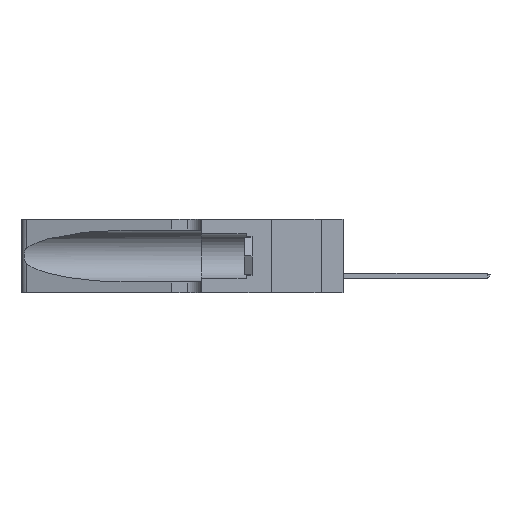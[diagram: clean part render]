
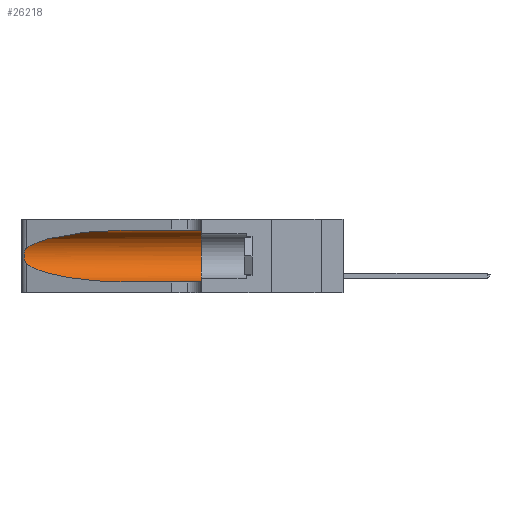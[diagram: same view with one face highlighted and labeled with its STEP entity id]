
A CAD part, left-side view. The second image highlights one B-rep face of the part: STEP entity #26218.
In plain terms, the highlighted cylindrical face has radius 3.308 mm (diameter 6.617 mm), a partial arc.
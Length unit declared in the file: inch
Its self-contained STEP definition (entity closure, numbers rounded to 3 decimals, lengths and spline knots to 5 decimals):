
#299 = LINE ( 'NONE', #27840, #22254 ) ;
#652 = CARTESIAN_POINT ( 'NONE',  ( 0.25487, 1.22718, 0.22369 ) ) ;
#789 = CARTESIAN_POINT ( 'NONE',  ( 0.25854, 1.2359, 0.20912 ) ) ;
#1079 = CARTESIAN_POINT ( 'NONE',  ( 0.25789, 1.23486, 0.15765 ) ) ;
#1167 = EDGE_CURVE ( 'NONE', #31608, #3406, #10031, .T. ) ;
#2053 = CARTESIAN_POINT ( 'NONE',  ( 0.18966, 0.96281, 0.31525 ) ) ;
#2174 = VERTEX_POINT ( 'NONE', #25149 ) ;
#3406 = VERTEX_POINT ( 'NONE', #5205 ) ;
#3571 = LINE ( 'NONE', #37456, #24119 ) ;
#3622 = ORIENTED_EDGE ( 'NONE', *, *, #30223, .T. ) ;
#5205 = CARTESIAN_POINT ( 'NONE',  ( 0.25487, 1.22718, 0.22369 ) ) ;
#6838 = CARTESIAN_POINT ( 'NONE',  ( 0.26018, 1.23835, 0.19895 ) ) ;
#7117 = CARTESIAN_POINT ( 'NONE',  ( 0.25787, 1.23484, 0.2124 ) ) ;
#7829 = VERTEX_POINT ( 'NONE', #31679 ) ;
#9673 = DIRECTION ( 'NONE',  ( 0., 0., 1. ) ) ;
#10031 =( BOUNDED_CURVE ( )  B_SPLINE_CURVE ( 3, ( #25748, #2053, #31788, #22376 ),
 .UNSPECIFIED., .F., .F. ) 
 B_SPLINE_CURVE_WITH_KNOTS ( ( 4, 4 ),
 ( 1.5708, 2.84003 ),
 .UNSPECIFIED. ) 
 CURVE ( )  GEOMETRIC_REPRESENTATION_ITEM ( )  RATIONAL_B_SPLINE_CURVE ( ( 1., 0.87, 0.87, 1. ) ) 
 REPRESENTATION_ITEM ( '' )  );
#11301 = CARTESIAN_POINT ( 'NONE',  ( 0.1305, 0.72297, 0.31525 ) ) ;
#11397 = ORIENTED_EDGE ( 'NONE', *, *, #26656, .F. ) ;
#11988 = AXIS2_PLACEMENT_3D ( 'NONE', #27702, #15833, #18851 ) ;
#12249 = CARTESIAN_POINT ( 'NONE',  ( 0.1305, 0.35, 0.05475 ) ) ;
#12529 = EDGE_CURVE ( 'NONE', #31608, #7829, #3571, .T. ) ;
#12671 = CARTESIAN_POINT ( 'NONE',  ( 0.25487, 1.22718, 0.14631 ) ) ;
#13066 = CARTESIAN_POINT ( 'NONE',  ( 0.25639, 1.23184, 0.21858 ) ) ;
#13346 = ORIENTED_EDGE ( 'NONE', *, *, #20162, .T. ) ;
#15113 = VERTEX_POINT ( 'NONE', #12249 ) ;
#15776 = CARTESIAN_POINT ( 'NONE',  ( 0.25856, 1.23593, 0.16098 ) ) ;
#15833 = DIRECTION ( 'NONE',  ( 0., -1., 0. ) ) ;
#16363 = CARTESIAN_POINT ( 'NONE',  ( 0.25487, 1.22718, 0.14631 ) ) ;
#16800 = FACE_OUTER_BOUND ( 'NONE', #24280, .T. ) ;
#18458 = DIRECTION ( 'NONE',  ( 0., 1., 0. ) ) ;
#18851 = DIRECTION ( 'NONE',  ( 0., 0., -1. ) ) ;
#19059 = CARTESIAN_POINT ( 'NONE',  ( 0.25639, 1.23186, 0.15144 ) ) ;
#19532 = DIRECTION ( 'NONE',  ( 0., -1., 0. ) ) ;
#20162 = EDGE_CURVE ( 'NONE', #2174, #15113, #299, .T. ) ;
#20496 = AXIS2_PLACEMENT_3D ( 'NONE', #24338, #18458, #9673 ) ;
#21499 = CARTESIAN_POINT ( 'NONE',  ( 0.26017, 1.23833, 0.17102 ) ) ;
#21636 = CARTESIAN_POINT ( 'NONE',  ( 0.25555, 1.22993, 0.14849 ) ) ;
#22254 = VECTOR ( 'NONE', #36480, 39.37008 ) ;
#22376 = CARTESIAN_POINT ( 'NONE',  ( 0.25487, 1.22718, 0.22369 ) ) ;
#23088 = CARTESIAN_POINT ( 'NONE',  ( 0.1305, 0.72297, 0.05475 ) ) ;
#23258 = ORIENTED_EDGE ( 'NONE', *, *, #35990, .T. ) ;
#23389 = VERTEX_POINT ( 'NONE', #16363 ) ;
#24119 = VECTOR ( 'NONE', #19532, 39.37008 ) ;
#24149 = CIRCLE ( 'NONE', #20496, 0.13025 ) ;
#24280 = EDGE_LOOP ( 'NONE', ( #34813, #23258, #3622, #13346, #11397, #37127 ) ) ;
#24338 = CARTESIAN_POINT ( 'NONE',  ( 0.1305, 0.35, 0.185 ) ) ;
#24519 = CARTESIAN_POINT ( 'NONE',  ( 0.26075, 1.23896, 0.19203 ) ) ;
#25149 = CARTESIAN_POINT ( 'NONE',  ( 0.1305, 0.72297, 0.05475 ) ) ;
#25748 = CARTESIAN_POINT ( 'NONE',  ( 0.1305, 0.72297, 0.31525 ) ) ;
#26050 = CARTESIAN_POINT ( 'NONE',  ( 0.18966, 0.96281, 0.05475 ) ) ;
#26218 = ADVANCED_FACE ( 'NONE', ( #16800 ), #31743, .F. ) ;
#26656 = EDGE_CURVE ( 'NONE', #7829, #15113, #24149, .T. ) ;
#27702 = CARTESIAN_POINT ( 'NONE',  ( 0.1305, 1.61858, 0.185 ) ) ;
#27840 = CARTESIAN_POINT ( 'NONE',  ( 0.1305, 1.61858, 0.05475 ) ) ;
#30223 = EDGE_CURVE ( 'NONE', #23389, #2174, #37050, .T. ) ;
#30532 = CARTESIAN_POINT ( 'NONE',  ( 0.26075, 1.23896, 0.178 ) ) ;
#31608 = VERTEX_POINT ( 'NONE', #11301 ) ;
#31679 = CARTESIAN_POINT ( 'NONE',  ( 0.1305, 0.35, 0.31525 ) ) ;
#31743 = CYLINDRICAL_SURFACE ( 'NONE', #11988, 0.13025 ) ;
#31788 = CARTESIAN_POINT ( 'NONE',  ( 0.2373, 1.15595, 0.28018 ) ) ;
#31949 = CARTESIAN_POINT ( 'NONE',  ( 0.25487, 1.22718, 0.14631 ) ) ;
#34813 = ORIENTED_EDGE ( 'NONE', *, *, #1167, .T. ) ;
#35990 = EDGE_CURVE ( 'NONE', #3406, #23389, #37809, .T. ) ;
#36480 = DIRECTION ( 'NONE',  ( 0., -1., 0. ) ) ;
#36693 = CARTESIAN_POINT ( 'NONE',  ( 0.25555, 1.22994, 0.2215 ) ) ;
#37050 =( BOUNDED_CURVE ( )  B_SPLINE_CURVE ( 3, ( #31949, #37986, #26050, #23088 ),
 .UNSPECIFIED., .F., .T. ) 
 B_SPLINE_CURVE_WITH_KNOTS ( ( 4, 4 ),
 ( 3.44316, 4.71239 ),
 .UNSPECIFIED. ) 
 CURVE ( )  GEOMETRIC_REPRESENTATION_ITEM ( )  RATIONAL_B_SPLINE_CURVE ( ( 1., 0.87, 0.87, 1. ) ) 
 REPRESENTATION_ITEM ( '' )  );
#37127 = ORIENTED_EDGE ( 'NONE', *, *, #12529, .F. ) ;
#37456 = CARTESIAN_POINT ( 'NONE',  ( 0.1305, 1.61858, 0.31525 ) ) ;
#37809 = B_SPLINE_CURVE_WITH_KNOTS ( 'NONE', 3,
 ( #652, #36693, #13066, #7117, #789, #6838, #24519, #30532, #21499, #15776, #1079, #19059, #21636, #12671 ),
 .UNSPECIFIED., .F., .F.,
 ( 4, 2, 2, 2, 2, 2, 4 ),
 ( 0., 0.00027, 0.00053, 0.00107, 0.0016, 0.00187, 0.00214 ),
 .UNSPECIFIED. ) ;
#37986 = CARTESIAN_POINT ( 'NONE',  ( 0.2373, 1.15595, 0.08982 ) ) ;
